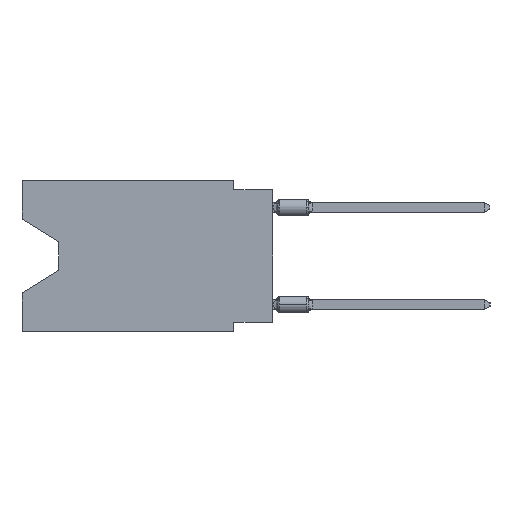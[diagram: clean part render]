
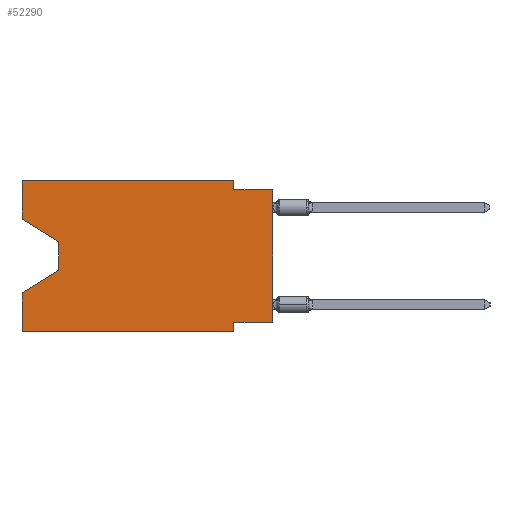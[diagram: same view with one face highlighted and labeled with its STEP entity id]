
A CAD part, left-side view. The second image highlights one B-rep face of the part: STEP entity #52290.
In plain terms, the highlighted planar face has unit normal (-1, 0, 0).
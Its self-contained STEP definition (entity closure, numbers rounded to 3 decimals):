
#591 = CARTESIAN_POINT ( 'NONE',  ( 0., 13.97, -5.893 ) ) ;
#2295 = EDGE_CURVE ( 'NONE', #39584, #18828, #38408, .T. ) ;
#2983 = LINE ( 'NONE', #7647, #34754 ) ;
#3771 = AXIS2_PLACEMENT_3D ( 'NONE', #57631, #10509, #14332 ) ;
#4678 = DIRECTION ( 'NONE',  ( 0., 0., -1. ) ) ;
#4960 = ORIENTED_EDGE ( 'NONE', *, *, #29848, .F. ) ;
#5520 = VECTOR ( 'NONE', #11490, 1000. ) ;
#6332 = VERTEX_POINT ( 'NONE', #23489 ) ;
#6466 = VECTOR ( 'NONE', #18801, 1000. ) ;
#6954 = DIRECTION ( 'NONE',  ( 0., -1., 0. ) ) ;
#7647 = CARTESIAN_POINT ( 'NONE',  ( 0., 16.383, 0. ) ) ;
#8489 = CARTESIAN_POINT ( 'NONE',  ( 0., 16.383, -2.546 ) ) ;
#9159 = ORIENTED_EDGE ( 'NONE', *, *, #2295, .F. ) ;
#9405 = DIRECTION ( 'NONE',  ( 0., 0., 1. ) ) ;
#10509 = DIRECTION ( 'NONE',  ( 1., 0., 0. ) ) ;
#11490 = DIRECTION ( 'NONE',  ( 0., 0., -1. ) ) ;
#12140 = VECTOR ( 'NONE', #18563, 1000. ) ;
#12544 = VERTEX_POINT ( 'NONE', #48997 ) ;
#12820 = EDGE_CURVE ( 'NONE', #55720, #18828, #49498, .T. ) ;
#12835 = ORIENTED_EDGE ( 'NONE', *, *, #54609, .F. ) ;
#13251 = CARTESIAN_POINT ( 'NONE',  ( 0., 13.97, -4.013 ) ) ;
#13371 = EDGE_CURVE ( 'NONE', #26164, #30977, #23362, .T. ) ;
#14297 = VECTOR ( 'NONE', #4678, 1000. ) ;
#14332 = DIRECTION ( 'NONE',  ( 0., 0., -1. ) ) ;
#16020 = VECTOR ( 'NONE', #40947, 1000. ) ;
#16054 = CARTESIAN_POINT ( 'NONE',  ( 0., 16.383, 0. ) ) ;
#16733 = VERTEX_POINT ( 'NONE', #13251 ) ;
#17760 = VERTEX_POINT ( 'NONE', #20497 ) ;
#17843 = DIRECTION ( 'NONE',  ( 0., -1., 0. ) ) ;
#17937 = EDGE_CURVE ( 'NONE', #23423, #16733, #57058, .T. ) ;
#18225 = DIRECTION ( 'NONE',  ( 0., 1., 0. ) ) ;
#18396 = VECTOR ( 'NONE', #17843, 1000. ) ;
#18563 = DIRECTION ( 'NONE',  ( 0., 0., -1. ) ) ;
#18801 = DIRECTION ( 'NONE',  ( 0., 0., 1. ) ) ;
#18828 = VERTEX_POINT ( 'NONE', #49312 ) ;
#18829 = CARTESIAN_POINT ( 'NONE',  ( 0., 2.54, -0.635 ) ) ;
#18984 = ORIENTED_EDGE ( 'NONE', *, *, #12820, .T. ) ;
#19412 = ORIENTED_EDGE ( 'NONE', *, *, #44022, .F. ) ;
#19870 = LINE ( 'NONE', #16054, #53405 ) ;
#20497 = CARTESIAN_POINT ( 'NONE',  ( 0., 16.383, -7.36 ) ) ;
#21420 = EDGE_CURVE ( 'NONE', #6332, #17760, #45347, .T. ) ;
#23362 = LINE ( 'NONE', #50016, #14297 ) ;
#23423 = VERTEX_POINT ( 'NONE', #44049 ) ;
#23489 = CARTESIAN_POINT ( 'NONE',  ( 0., 13.97, -5.893 ) ) ;
#24109 = EDGE_CURVE ( 'NONE', #12544, #17760, #50684, .T. ) ;
#24700 = EDGE_LOOP ( 'NONE', ( #26076, #42364, #29960, #35600, #43063, #40785, #12835, #18984, #9159, #26946, #19412, #4960 ) ) ;
#24934 = LINE ( 'NONE', #55094, #5520 ) ;
#26076 = ORIENTED_EDGE ( 'NONE', *, *, #17937, .T. ) ;
#26164 = VERTEX_POINT ( 'NONE', #29295 ) ;
#26313 = FACE_OUTER_BOUND ( 'NONE', #24700, .T. ) ;
#26367 = VERTEX_POINT ( 'NONE', #27784 ) ;
#26758 = VECTOR ( 'NONE', #26899, 1000. ) ;
#26899 = DIRECTION ( 'NONE',  ( 0., -0.855, -0.519 ) ) ;
#26946 = ORIENTED_EDGE ( 'NONE', *, *, #32887, .F. ) ;
#27250 = VECTOR ( 'NONE', #18225, 1000. ) ;
#27784 = CARTESIAN_POINT ( 'NONE',  ( 0., 2.54, 0. ) ) ;
#28267 = EDGE_CURVE ( 'NONE', #12544, #30977, #42644, .T. ) ;
#28730 = CARTESIAN_POINT ( 'NONE',  ( 0., 16.383, 0. ) ) ;
#28866 = CARTESIAN_POINT ( 'NONE',  ( 0., 16.383, -9.906 ) ) ;
#29295 = CARTESIAN_POINT ( 'NONE',  ( 0., 2.54, -9.271 ) ) ;
#29848 = EDGE_CURVE ( 'NONE', #23423, #32828, #2983, .T. ) ;
#29861 = DIRECTION ( 'NONE',  ( 0., 0., 1. ) ) ;
#29960 = ORIENTED_EDGE ( 'NONE', *, *, #21420, .T. ) ;
#30977 = VERTEX_POINT ( 'NONE', #49925 ) ;
#31428 = CARTESIAN_POINT ( 'NONE',  ( 0., 13.97, -4.013 ) ) ;
#32828 = VERTEX_POINT ( 'NONE', #28730 ) ;
#32887 = EDGE_CURVE ( 'NONE', #26367, #39584, #24934, .T. ) ;
#34754 = VECTOR ( 'NONE', #29861, 1000. ) ;
#35600 = ORIENTED_EDGE ( 'NONE', *, *, #24109, .F. ) ;
#38339 = VECTOR ( 'NONE', #6954, 1000. ) ;
#38408 = LINE ( 'NONE', #51605, #18396 ) ;
#39584 = VERTEX_POINT ( 'NONE', #18829 ) ;
#40148 = CARTESIAN_POINT ( 'NONE',  ( 0., 0., -9.271 ) ) ;
#40785 = ORIENTED_EDGE ( 'NONE', *, *, #13371, .F. ) ;
#40947 = DIRECTION ( 'NONE',  ( 0., 0.855, -0.519 ) ) ;
#42177 = VECTOR ( 'NONE', #9405, 1000. ) ;
#42364 = ORIENTED_EDGE ( 'NONE', *, *, #52696, .T. ) ;
#42644 = LINE ( 'NONE', #28866, #38339 ) ;
#43063 = ORIENTED_EDGE ( 'NONE', *, *, #28267, .T. ) ;
#43269 = DIRECTION ( 'NONE',  ( 0., -1., 0. ) ) ;
#44022 = EDGE_CURVE ( 'NONE', #32828, #26367, #19870, .T. ) ;
#44049 = CARTESIAN_POINT ( 'NONE',  ( 0., 16.383, -2.546 ) ) ;
#44186 = PLANE ( 'NONE',  #3771 ) ;
#44554 = LINE ( 'NONE', #40148, #27250 ) ;
#44812 = CARTESIAN_POINT ( 'NONE',  ( 0., 0., 0. ) ) ;
#45347 = LINE ( 'NONE', #591, #16020 ) ;
#45764 = LINE ( 'NONE', #31428, #12140 ) ;
#47588 = CARTESIAN_POINT ( 'NONE',  ( 0., 0., -9.271 ) ) ;
#48997 = CARTESIAN_POINT ( 'NONE',  ( 0., 16.383, -9.906 ) ) ;
#49312 = CARTESIAN_POINT ( 'NONE',  ( 0., 0., -0.635 ) ) ;
#49498 = LINE ( 'NONE', #44812, #42177 ) ;
#49925 = CARTESIAN_POINT ( 'NONE',  ( 0., 2.54, -9.906 ) ) ;
#50016 = CARTESIAN_POINT ( 'NONE',  ( 0., 2.54, -9.906 ) ) ;
#50684 = LINE ( 'NONE', #54513, #6466 ) ;
#51605 = CARTESIAN_POINT ( 'NONE',  ( 0., 0., -0.635 ) ) ;
#52290 = ADVANCED_FACE ( 'NONE', ( #26313 ), #44186, .F. ) ;
#52696 = EDGE_CURVE ( 'NONE', #16733, #6332, #45764, .T. ) ;
#53405 = VECTOR ( 'NONE', #43269, 1000. ) ;
#54513 = CARTESIAN_POINT ( 'NONE',  ( 0., 16.383, 0. ) ) ;
#54609 = EDGE_CURVE ( 'NONE', #55720, #26164, #44554, .T. ) ;
#55094 = CARTESIAN_POINT ( 'NONE',  ( 0., 2.54, 0. ) ) ;
#55720 = VERTEX_POINT ( 'NONE', #47588 ) ;
#57058 = LINE ( 'NONE', #8489, #26758 ) ;
#57631 = CARTESIAN_POINT ( 'NONE',  ( 0., 16.383, 0. ) ) ;
